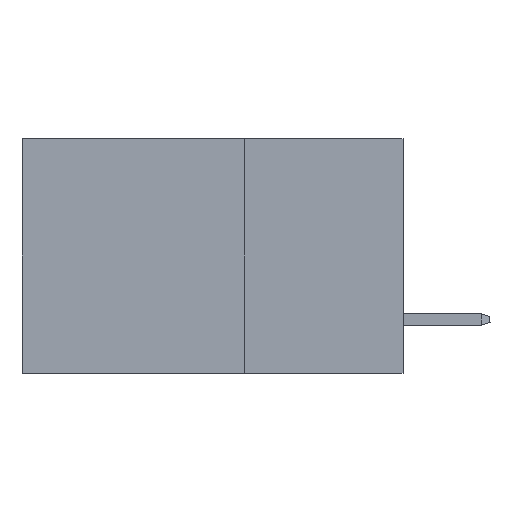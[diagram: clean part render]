
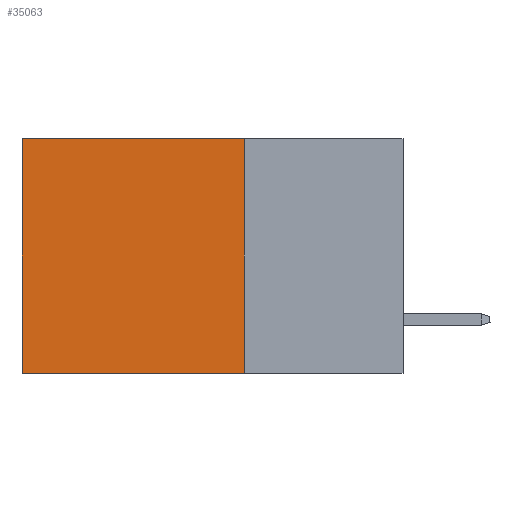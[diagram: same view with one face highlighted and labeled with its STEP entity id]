
A CAD part, left-side view. The second image highlights one B-rep face of the part: STEP entity #35063.
In plain terms, the highlighted planar face has unit normal (-1, 0, 0).
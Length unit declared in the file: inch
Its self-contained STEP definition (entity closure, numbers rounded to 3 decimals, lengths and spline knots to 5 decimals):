
#39 = VECTOR ( 'NONE', #4826, 39.37008 ) ;
#1605 = DIRECTION ( 'NONE',  ( 0., 0., -1. ) ) ;
#1638 = CARTESIAN_POINT ( 'NONE',  ( 0.2875, 0.25, 0. ) ) ;
#1768 = ORIENTED_EDGE ( 'NONE', *, *, #30156, .T. ) ;
#3358 = VECTOR ( 'NONE', #14983, 39.37008 ) ;
#4826 = DIRECTION ( 'NONE',  ( 0., 1., 0. ) ) ;
#5644 = VERTEX_POINT ( 'NONE', #24754 ) ;
#6711 = DIRECTION ( 'NONE',  ( 1., 0., 0. ) ) ;
#7850 = LINE ( 'NONE', #24604, #16180 ) ;
#8417 = VECTOR ( 'NONE', #21091, 39.37008 ) ;
#8516 = LINE ( 'NONE', #19613, #3358 ) ;
#9542 = EDGE_CURVE ( 'NONE', #33914, #20343, #8516, .T. ) ;
#10130 = CARTESIAN_POINT ( 'NONE',  ( 0.2875, 0.25, 0. ) ) ;
#10606 = LINE ( 'NONE', #29739, #39 ) ;
#10648 = CARTESIAN_POINT ( 'NONE',  ( 0.2875, 0.25, 0. ) ) ;
#11369 = VERTEX_POINT ( 'NONE', #18580 ) ;
#11414 = EDGE_CURVE ( 'NONE', #5644, #11369, #7850, .T. ) ;
#14983 = DIRECTION ( 'NONE',  ( 0., 0., -1. ) ) ;
#16180 = VECTOR ( 'NONE', #21674, 39.37008 ) ;
#17803 = ORIENTED_EDGE ( 'NONE', *, *, #9542, .F. ) ;
#18580 = CARTESIAN_POINT ( 'NONE',  ( 0.2875, 0.6, -0.37 ) ) ;
#19613 = CARTESIAN_POINT ( 'NONE',  ( 0.2875, 0.25, 0. ) ) ;
#20302 = ORIENTED_EDGE ( 'NONE', *, *, #25482, .F. ) ;
#20343 = VERTEX_POINT ( 'NONE', #27034 ) ;
#21091 = DIRECTION ( 'NONE',  ( 0., 1., 0. ) ) ;
#21514 = AXIS2_PLACEMENT_3D ( 'NONE', #10130, #6711, #1605 ) ;
#21674 = DIRECTION ( 'NONE',  ( 0., 0., -1. ) ) ;
#24155 = EDGE_LOOP ( 'NONE', ( #31632, #20302, #17803, #1768 ) ) ;
#24604 = CARTESIAN_POINT ( 'NONE',  ( 0.2875, 0.6, 0. ) ) ;
#24754 = CARTESIAN_POINT ( 'NONE',  ( 0.2875, 0.6, 0. ) ) ;
#25482 = EDGE_CURVE ( 'NONE', #20343, #11369, #10606, .T. ) ;
#26527 = FACE_OUTER_BOUND ( 'NONE', #24155, .T. ) ;
#26552 = LINE ( 'NONE', #1638, #8417 ) ;
#27034 = CARTESIAN_POINT ( 'NONE',  ( 0.2875, 0.25, -0.37 ) ) ;
#29739 = CARTESIAN_POINT ( 'NONE',  ( 0.2875, 0.25, -0.37 ) ) ;
#30156 = EDGE_CURVE ( 'NONE', #33914, #5644, #26552, .T. ) ;
#31632 = ORIENTED_EDGE ( 'NONE', *, *, #11414, .T. ) ;
#31660 = PLANE ( 'NONE',  #21514 ) ;
#33914 = VERTEX_POINT ( 'NONE', #10648 ) ;
#35063 = ADVANCED_FACE ( 'NONE', ( #26527 ), #31660, .F. ) ;
